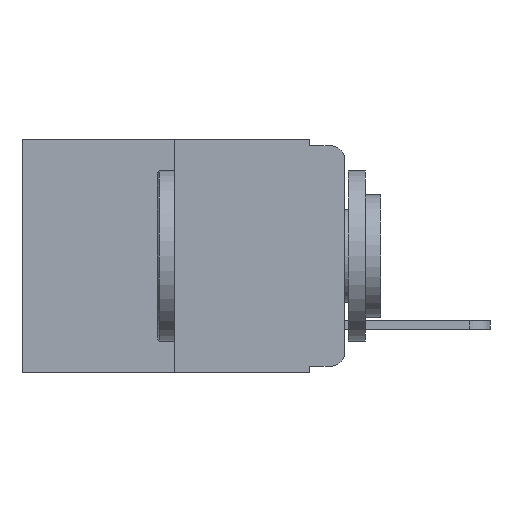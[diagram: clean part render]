
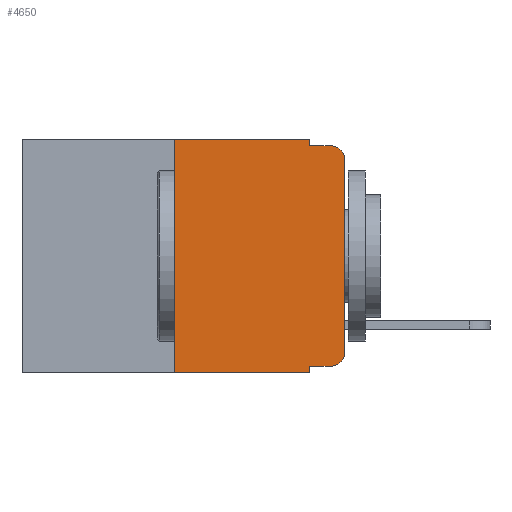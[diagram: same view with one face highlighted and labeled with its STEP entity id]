
A CAD part, left-side view. The second image highlights one B-rep face of the part: STEP entity #4650.
In plain terms, the highlighted planar face has unit normal (-1, 0, 0).
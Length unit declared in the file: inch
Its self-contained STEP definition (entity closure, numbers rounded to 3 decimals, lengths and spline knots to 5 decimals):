
#462 = CARTESIAN_POINT ( 'NONE',  ( 0., 0., -0.03 ) ) ;
#541 = VERTEX_POINT ( 'NONE', #18910 ) ;
#605 = EDGE_LOOP ( 'NONE', ( #8506, #17030, #16093, #4991, #14812, #12910, #17559, #11650, #8325, #8889 ) ) ;
#952 = CARTESIAN_POINT ( 'NONE',  ( 0., 0.051, 0. ) ) ;
#981 = EDGE_CURVE ( 'NONE', #9328, #5993, #14508, .T. ) ;
#1056 = LINE ( 'NONE', #9605, #19148 ) ;
#1100 = CARTESIAN_POINT ( 'NONE',  ( 0., 0., -0.313 ) ) ;
#1161 = VECTOR ( 'NONE', #8606, 39.37008 ) ;
#1649 = DIRECTION ( 'NONE',  ( 0., 0., -1. ) ) ;
#2762 = EDGE_CURVE ( 'NONE', #14027, #15017, #21105, .T. ) ;
#2886 = CARTESIAN_POINT ( 'NONE',  ( 0., 0.051, -0.01 ) ) ;
#3763 = CIRCLE ( 'NONE', #8058, 0.02 ) ;
#3909 = CARTESIAN_POINT ( 'NONE',  ( 0., 0.051, -0.333 ) ) ;
#4062 = CARTESIAN_POINT ( 'NONE',  ( 0., 0.051, 0. ) ) ;
#4650 = ADVANCED_FACE ( 'NONE', ( #16981 ), #20042, .F. ) ;
#4991 = ORIENTED_EDGE ( 'NONE', *, *, #8564, .F. ) ;
#5228 = EDGE_CURVE ( 'NONE', #541, #11159, #1056, .T. ) ;
#5789 = DIRECTION ( 'NONE',  ( 0., 0., -1. ) ) ;
#5993 = VERTEX_POINT ( 'NONE', #7308 ) ;
#6123 = VECTOR ( 'NONE', #11541, 39.37008 ) ;
#6623 = EDGE_CURVE ( 'NONE', #11063, #9328, #13337, .T. ) ;
#6672 = EDGE_CURVE ( 'NONE', #14027, #11159, #14993, .T. ) ;
#6674 = VERTEX_POINT ( 'NONE', #8519 ) ;
#6722 = LINE ( 'NONE', #11697, #6123 ) ;
#6848 = LINE ( 'NONE', #952, #15433 ) ;
#7308 = CARTESIAN_POINT ( 'NONE',  ( 0., 0.02, -0.01 ) ) ;
#7450 = EDGE_CURVE ( 'NONE', #10969, #5993, #18932, .T. ) ;
#7761 = DIRECTION ( 'NONE',  ( -1., 0., 0. ) ) ;
#8058 = AXIS2_PLACEMENT_3D ( 'NONE', #17331, #7761, #18913 ) ;
#8325 = ORIENTED_EDGE ( 'NONE', *, *, #2762, .T. ) ;
#8506 = ORIENTED_EDGE ( 'NONE', *, *, #6623, .T. ) ;
#8519 = CARTESIAN_POINT ( 'NONE',  ( 0., 0.25, 0. ) ) ;
#8564 = EDGE_CURVE ( 'NONE', #16716, #10969, #6848, .T. ) ;
#8606 = DIRECTION ( 'NONE',  ( 0., 0., -1. ) ) ;
#8704 = CARTESIAN_POINT ( 'NONE',  ( 0., 0.051, 0. ) ) ;
#8889 = ORIENTED_EDGE ( 'NONE', *, *, #18943, .T. ) ;
#9155 = CARTESIAN_POINT ( 'NONE',  ( 0., 0.473, 0. ) ) ;
#9328 = VERTEX_POINT ( 'NONE', #462 ) ;
#9545 = DIRECTION ( 'NONE',  ( 0., -1., 0. ) ) ;
#9574 = CARTESIAN_POINT ( 'NONE',  ( 0., 0., 0. ) ) ;
#9605 = CARTESIAN_POINT ( 'NONE',  ( 0., 0.473, -0.343 ) ) ;
#9685 = AXIS2_PLACEMENT_3D ( 'NONE', #20290, #19997, #19974 ) ;
#9686 = DIRECTION ( 'NONE',  ( 0., 0., 1. ) ) ;
#10524 = VECTOR ( 'NONE', #18476, 39.37008 ) ;
#10831 = DIRECTION ( 'NONE',  ( 0., -1., 0. ) ) ;
#10969 = VERTEX_POINT ( 'NONE', #2886 ) ;
#11063 = VERTEX_POINT ( 'NONE', #1100 ) ;
#11159 = VERTEX_POINT ( 'NONE', #20591 ) ;
#11541 = DIRECTION ( 'NONE',  ( 0., 0., 1. ) ) ;
#11650 = ORIENTED_EDGE ( 'NONE', *, *, #6672, .F. ) ;
#11697 = CARTESIAN_POINT ( 'NONE',  ( 0., 0.25, 0. ) ) ;
#11750 = DIRECTION ( 'NONE',  ( -1., 0., 0. ) ) ;
#12256 = EDGE_CURVE ( 'NONE', #541, #6674, #6722, .T. ) ;
#12910 = ORIENTED_EDGE ( 'NONE', *, *, #12256, .F. ) ;
#12963 = VECTOR ( 'NONE', #17233, 39.37008 ) ;
#13337 = LINE ( 'NONE', #9574, #21009 ) ;
#14027 = VERTEX_POINT ( 'NONE', #3909 ) ;
#14508 = CIRCLE ( 'NONE', #16522, 0.02 ) ;
#14812 = ORIENTED_EDGE ( 'NONE', *, *, #21642, .F. ) ;
#14993 = LINE ( 'NONE', #8704, #1161 ) ;
#15017 = VERTEX_POINT ( 'NONE', #15805 ) ;
#15433 = VECTOR ( 'NONE', #1649, 39.37008 ) ;
#15805 = CARTESIAN_POINT ( 'NONE',  ( 0., 0.02, -0.333 ) ) ;
#15850 = CARTESIAN_POINT ( 'NONE',  ( 0., 0.051, -0.333 ) ) ;
#16093 = ORIENTED_EDGE ( 'NONE', *, *, #7450, .F. ) ;
#16522 = AXIS2_PLACEMENT_3D ( 'NONE', #18959, #11750, #5789 ) ;
#16716 = VERTEX_POINT ( 'NONE', #4062 ) ;
#16906 = VECTOR ( 'NONE', #10831, 39.37008 ) ;
#16981 = FACE_OUTER_BOUND ( 'NONE', #605, .T. ) ;
#17030 = ORIENTED_EDGE ( 'NONE', *, *, #981, .T. ) ;
#17233 = DIRECTION ( 'NONE',  ( 0., -1., 0. ) ) ;
#17331 = CARTESIAN_POINT ( 'NONE',  ( 0., 0.02, -0.313 ) ) ;
#17559 = ORIENTED_EDGE ( 'NONE', *, *, #5228, .T. ) ;
#18476 = DIRECTION ( 'NONE',  ( 0., -1., 0. ) ) ;
#18910 = CARTESIAN_POINT ( 'NONE',  ( 0., 0.25, -0.343 ) ) ;
#18913 = DIRECTION ( 'NONE',  ( 0., 0., -1. ) ) ;
#18932 = LINE ( 'NONE', #19089, #10524 ) ;
#18943 = EDGE_CURVE ( 'NONE', #15017, #11063, #3763, .T. ) ;
#18959 = CARTESIAN_POINT ( 'NONE',  ( 0., 0.02, -0.03 ) ) ;
#19089 = CARTESIAN_POINT ( 'NONE',  ( 0., 0.051, -0.01 ) ) ;
#19148 = VECTOR ( 'NONE', #9545, 39.37008 ) ;
#19974 = DIRECTION ( 'NONE',  ( 0., 0., -1. ) ) ;
#19997 = DIRECTION ( 'NONE',  ( 1., 0., 0. ) ) ;
#20042 = PLANE ( 'NONE',  #9685 ) ;
#20290 = CARTESIAN_POINT ( 'NONE',  ( 0., 0.473, 0. ) ) ;
#20591 = CARTESIAN_POINT ( 'NONE',  ( 0., 0.051, -0.343 ) ) ;
#20913 = LINE ( 'NONE', #9155, #16906 ) ;
#21009 = VECTOR ( 'NONE', #9686, 39.37008 ) ;
#21105 = LINE ( 'NONE', #15850, #12963 ) ;
#21642 = EDGE_CURVE ( 'NONE', #6674, #16716, #20913, .T. ) ;
